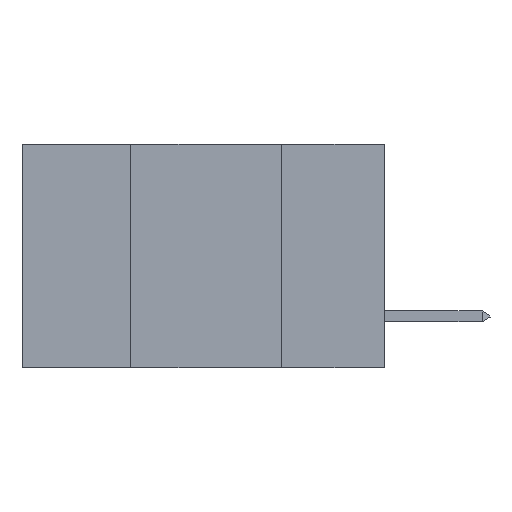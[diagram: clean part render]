
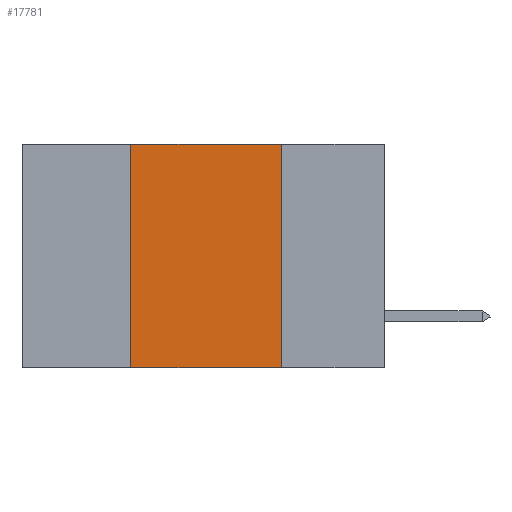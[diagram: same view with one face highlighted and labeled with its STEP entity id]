
A CAD part, left-side view. The second image highlights one B-rep face of the part: STEP entity #17781.
In plain terms, the highlighted planar face has unit normal (-1, 0, 0).
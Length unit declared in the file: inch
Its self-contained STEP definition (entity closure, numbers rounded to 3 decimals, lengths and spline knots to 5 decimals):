
#412 = DIRECTION ( 'NONE',  ( 0., 0., -1. ) ) ;
#471 = CARTESIAN_POINT ( 'NONE',  ( 0., 0.17, -0.37 ) ) ;
#1870 = ORIENTED_EDGE ( 'NONE', *, *, #31464, .T. ) ;
#5935 = DIRECTION ( 'NONE',  ( 1., 0., 0. ) ) ;
#6235 = CARTESIAN_POINT ( 'NONE',  ( 0., 0.6, -0.37 ) ) ;
#7100 = CARTESIAN_POINT ( 'NONE',  ( 0., 0.6, 0. ) ) ;
#10798 = LINE ( 'NONE', #7100, #16265 ) ;
#11052 = DIRECTION ( 'NONE',  ( 0., -1., 0. ) ) ;
#11491 = FACE_OUTER_BOUND ( 'NONE', #27951, .T. ) ;
#11980 = ORIENTED_EDGE ( 'NONE', *, *, #29606, .F. ) ;
#14638 = AXIS2_PLACEMENT_3D ( 'NONE', #25047, #5935, #29946 ) ;
#15541 = CARTESIAN_POINT ( 'NONE',  ( 0., 0.42, 0. ) ) ;
#16179 = VERTEX_POINT ( 'NONE', #23488 ) ;
#16265 = VECTOR ( 'NONE', #32404, 39.37008 ) ;
#16640 = DIRECTION ( 'NONE',  ( 0., 0., 1. ) ) ;
#17781 = ADVANCED_FACE ( 'NONE', ( #11491 ), #27255, .F. ) ;
#22012 = LINE ( 'NONE', #29850, #31247 ) ;
#22045 = EDGE_CURVE ( 'NONE', #31194, #16179, #10798, .T. ) ;
#22347 = VECTOR ( 'NONE', #16640, 39.37008 ) ;
#22550 = ORIENTED_EDGE ( 'NONE', *, *, #30796, .F. ) ;
#23488 = CARTESIAN_POINT ( 'NONE',  ( 0., 0.17, 0. ) ) ;
#23981 = LINE ( 'NONE', #6235, #31949 ) ;
#25047 = CARTESIAN_POINT ( 'NONE',  ( 0., 0.6, 0. ) ) ;
#27255 = PLANE ( 'NONE',  #14638 ) ;
#27951 = EDGE_LOOP ( 'NONE', ( #11980, #34534, #22550, #1870 ) ) ;
#29606 = EDGE_CURVE ( 'NONE', #16179, #32696, #22012, .T. ) ;
#29850 = CARTESIAN_POINT ( 'NONE',  ( 0., 0.17, 0. ) ) ;
#29946 = DIRECTION ( 'NONE',  ( 0., 0., -1. ) ) ;
#30325 = LINE ( 'NONE', #32759, #22347 ) ;
#30796 = EDGE_CURVE ( 'NONE', #34780, #31194, #30325, .T. ) ;
#30937 = CARTESIAN_POINT ( 'NONE',  ( 0., 0.42, -0.37 ) ) ;
#31194 = VERTEX_POINT ( 'NONE', #15541 ) ;
#31247 = VECTOR ( 'NONE', #412, 39.37008 ) ;
#31464 = EDGE_CURVE ( 'NONE', #34780, #32696, #23981, .T. ) ;
#31949 = VECTOR ( 'NONE', #11052, 39.37008 ) ;
#32404 = DIRECTION ( 'NONE',  ( 0., -1., 0. ) ) ;
#32696 = VERTEX_POINT ( 'NONE', #471 ) ;
#32759 = CARTESIAN_POINT ( 'NONE',  ( 0., 0.42, 0. ) ) ;
#34534 = ORIENTED_EDGE ( 'NONE', *, *, #22045, .F. ) ;
#34780 = VERTEX_POINT ( 'NONE', #30937 ) ;
